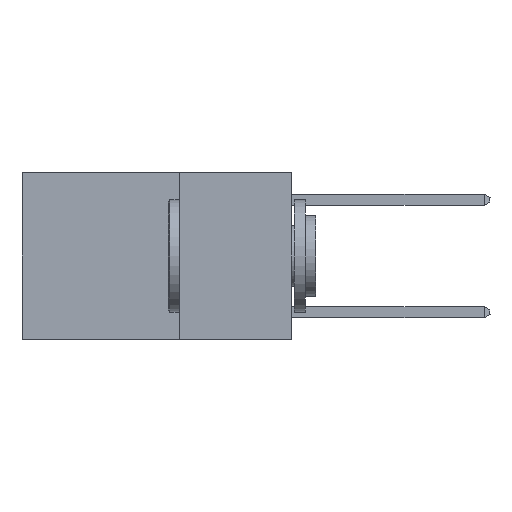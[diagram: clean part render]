
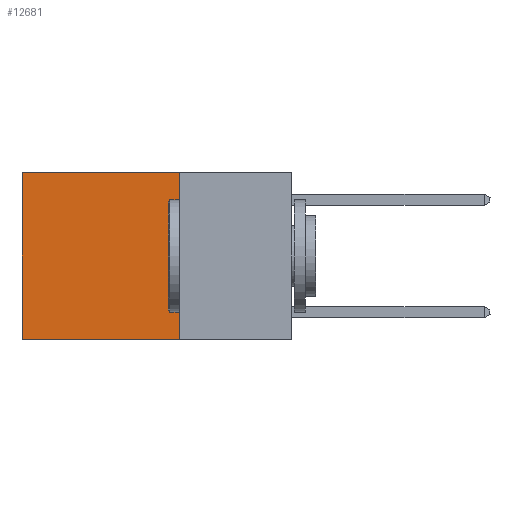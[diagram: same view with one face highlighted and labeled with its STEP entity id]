
A CAD part, left-side view. The second image highlights one B-rep face of the part: STEP entity #12681.
In plain terms, the highlighted planar face has unit normal (-1, 0, 0).
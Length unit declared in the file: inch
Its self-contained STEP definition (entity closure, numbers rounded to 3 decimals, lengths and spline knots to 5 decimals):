
#43 = DIRECTION ( 'NONE',  ( 0., 0., -1. ) ) ;
#1671 = EDGE_CURVE ( 'NONE', #4902, #19422, #24638, .T. ) ;
#1798 = EDGE_CURVE ( 'NONE', #8109, #19422, #23393, .T. ) ;
#2278 = ORIENTED_EDGE ( 'NONE', *, *, #11018, .F. ) ;
#2364 = VERTEX_POINT ( 'NONE', #22829 ) ;
#2454 = VECTOR ( 'NONE', #6064, 39.37008 ) ;
#2955 = DIRECTION ( 'NONE',  ( 0., 0., -1. ) ) ;
#3125 = DIRECTION ( 'NONE',  ( 0., 0., -1. ) ) ;
#4902 = VERTEX_POINT ( 'NONE', #12651 ) ;
#5626 = DIRECTION ( 'NONE',  ( 0., 1., 0. ) ) ;
#5994 = CARTESIAN_POINT ( 'NONE',  ( 0.2625, 0.25, 0. ) ) ;
#6064 = DIRECTION ( 'NONE',  ( 0., 1., 0. ) ) ;
#6180 = AXIS2_PLACEMENT_3D ( 'NONE', #20252, #17847, #2955 ) ;
#6730 = FACE_OUTER_BOUND ( 'NONE', #20438, .T. ) ;
#6893 = CARTESIAN_POINT ( 'NONE',  ( 0.2625, 0.25, 0. ) ) ;
#8109 = VERTEX_POINT ( 'NONE', #23607 ) ;
#9808 = EDGE_CURVE ( 'NONE', #2364, #4902, #17007, .T. ) ;
#10423 = VECTOR ( 'NONE', #3125, 39.37008 ) ;
#11018 = EDGE_CURVE ( 'NONE', #2364, #8109, #18639, .T. ) ;
#12651 = CARTESIAN_POINT ( 'NONE',  ( 0.2625, 0.6, 0. ) ) ;
#12681 = ADVANCED_FACE ( 'NONE', ( #6730 ), #19736, .F. ) ;
#12810 = VECTOR ( 'NONE', #5626, 39.37008 ) ;
#13900 = ORIENTED_EDGE ( 'NONE', *, *, #1798, .F. ) ;
#14732 = CARTESIAN_POINT ( 'NONE',  ( 0.2625, 0.6, -0.37 ) ) ;
#17007 = LINE ( 'NONE', #5994, #12810 ) ;
#17314 = ORIENTED_EDGE ( 'NONE', *, *, #9808, .T. ) ;
#17329 = CARTESIAN_POINT ( 'NONE',  ( 0.2625, 0.6, 0. ) ) ;
#17823 = CARTESIAN_POINT ( 'NONE',  ( 0.2625, 0.25, -0.37 ) ) ;
#17847 = DIRECTION ( 'NONE',  ( 1., 0., 0. ) ) ;
#18639 = LINE ( 'NONE', #6893, #10423 ) ;
#19422 = VERTEX_POINT ( 'NONE', #14732 ) ;
#19736 = PLANE ( 'NONE',  #6180 ) ;
#20252 = CARTESIAN_POINT ( 'NONE',  ( 0.2625, 0.25, 0. ) ) ;
#20438 = EDGE_LOOP ( 'NONE', ( #24841, #13900, #2278, #17314 ) ) ;
#22829 = CARTESIAN_POINT ( 'NONE',  ( 0.2625, 0.25, 0. ) ) ;
#23393 = LINE ( 'NONE', #17823, #2454 ) ;
#23418 = VECTOR ( 'NONE', #43, 39.37008 ) ;
#23607 = CARTESIAN_POINT ( 'NONE',  ( 0.2625, 0.25, -0.37 ) ) ;
#24638 = LINE ( 'NONE', #17329, #23418 ) ;
#24841 = ORIENTED_EDGE ( 'NONE', *, *, #1671, .T. ) ;
